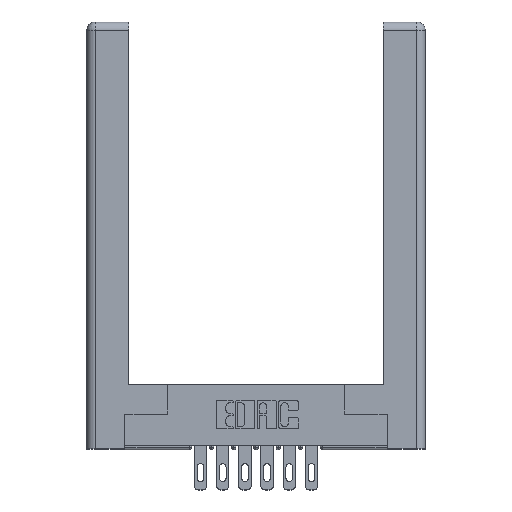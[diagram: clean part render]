
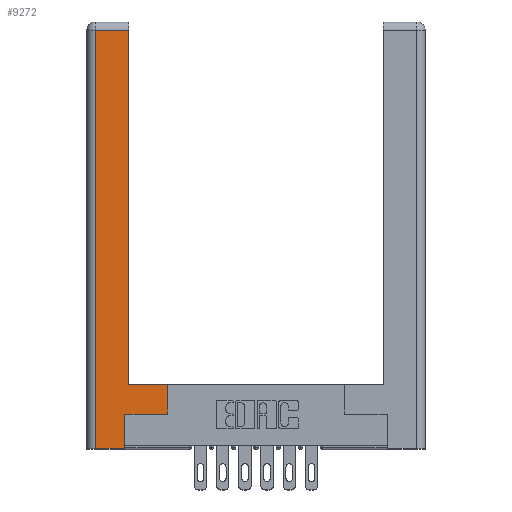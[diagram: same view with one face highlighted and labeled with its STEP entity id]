
A CAD part, top view. The second image highlights one B-rep face of the part: STEP entity #9272.
In plain terms, the highlighted planar face has unit normal (0, 0, 1).
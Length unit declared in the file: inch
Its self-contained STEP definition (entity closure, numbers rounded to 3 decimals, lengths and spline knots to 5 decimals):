
#87 = ORIENTED_EDGE ( 'NONE', *, *, #5223, .T. ) ;
#335 = ORIENTED_EDGE ( 'NONE', *, *, #5017, .T. ) ;
#490 = VECTOR ( 'NONE', #10808, 39.37008 ) ;
#1028 = CARTESIAN_POINT ( 'NONE',  ( 0.295, 3., 0. ) ) ;
#1227 = VECTOR ( 'NONE', #6869, 39.37008 ) ;
#1341 = CARTESIAN_POINT ( 'NONE',  ( 0.265, 0., 0. ) ) ;
#2209 = CARTESIAN_POINT ( 'NONE',  ( 0.0615, 0., 0. ) ) ;
#2702 = ORIENTED_EDGE ( 'NONE', *, *, #5107, .T. ) ;
#2739 = CARTESIAN_POINT ( 'NONE',  ( 0.565, 0.245, 0. ) ) ;
#3111 = CARTESIAN_POINT ( 'NONE',  ( 0.295, 0.45, 0. ) ) ;
#3531 = LINE ( 'NONE', #10332, #490 ) ;
#3705 = CARTESIAN_POINT ( 'NONE',  ( 0.295, 0.45, 0. ) ) ;
#3775 = LINE ( 'NONE', #5520, #8857 ) ;
#3804 = CARTESIAN_POINT ( 'NONE',  ( 0.0615, 2.94, 0. ) ) ;
#3820 = VERTEX_POINT ( 'NONE', #2209 ) ;
#3866 = FACE_OUTER_BOUND ( 'NONE', #8218, .T. ) ;
#4005 = VERTEX_POINT ( 'NONE', #3705 ) ;
#4191 = ORIENTED_EDGE ( 'NONE', *, *, #7445, .T. ) ;
#4548 = DIRECTION ( 'NONE',  ( -1., 0., 0. ) ) ;
#4716 = CARTESIAN_POINT ( 'NONE',  ( 0.295, 2.94, 0. ) ) ;
#4779 = AXIS2_PLACEMENT_3D ( 'NONE', #11039, #10870, #10853 ) ;
#5017 = EDGE_CURVE ( 'NONE', #3820, #8410, #3531, .T. ) ;
#5107 = EDGE_CURVE ( 'NONE', #12097, #4005, #12753, .T. ) ;
#5155 = VECTOR ( 'NONE', #4548, 39.37008 ) ;
#5193 = VERTEX_POINT ( 'NONE', #4716 ) ;
#5223 = EDGE_CURVE ( 'NONE', #4005, #5193, #8110, .T. ) ;
#5245 = EDGE_CURVE ( 'NONE', #5193, #6784, #10182, .T. ) ;
#5520 = CARTESIAN_POINT ( 'NONE',  ( 0.265, 0.245, 0. ) ) ;
#5847 = ORIENTED_EDGE ( 'NONE', *, *, #5245, .T. ) ;
#6556 = DIRECTION ( 'NONE',  ( 0., 1., 0. ) ) ;
#6784 = VERTEX_POINT ( 'NONE', #10791 ) ;
#6869 = DIRECTION ( 'NONE',  ( 1., 0., 0. ) ) ;
#6936 = VERTEX_POINT ( 'NONE', #6988 ) ;
#6988 = CARTESIAN_POINT ( 'NONE',  ( 0.565, 0.245, 0. ) ) ;
#7052 = VECTOR ( 'NONE', #7135, 39.37008 ) ;
#7135 = DIRECTION ( 'NONE',  ( 0., -1., 0. ) ) ;
#7342 = VECTOR ( 'NONE', #11834, 39.37008 ) ;
#7445 = EDGE_CURVE ( 'NONE', #6936, #12097, #12194, .T. ) ;
#7463 = CARTESIAN_POINT ( 'NONE',  ( 0.0615, 0., 0. ) ) ;
#8048 = ORIENTED_EDGE ( 'NONE', *, *, #9053, .T. ) ;
#8110 = LINE ( 'NONE', #1028, #12854 ) ;
#8218 = EDGE_LOOP ( 'NONE', ( #87, #5847, #8048, #335, #9637, #10563, #4191, #2702 ) ) ;
#8410 = VERTEX_POINT ( 'NONE', #1341 ) ;
#8743 = VERTEX_POINT ( 'NONE', #9324 ) ;
#8757 = CARTESIAN_POINT ( 'NONE',  ( 0.565, 0.45, 0. ) ) ;
#8857 = VECTOR ( 'NONE', #6556, 39.37008 ) ;
#9053 = EDGE_CURVE ( 'NONE', #6784, #3820, #9699, .T. ) ;
#9256 = LINE ( 'NONE', #2739, #1227 ) ;
#9272 = ADVANCED_FACE ( 'NONE', ( #3866 ), #10915, .F. ) ;
#9324 = CARTESIAN_POINT ( 'NONE',  ( 0.265, 0.245, 0. ) ) ;
#9637 = ORIENTED_EDGE ( 'NONE', *, *, #11997, .T. ) ;
#9699 = LINE ( 'NONE', #7463, #7052 ) ;
#10097 = EDGE_CURVE ( 'NONE', #8743, #6936, #9256, .T. ) ;
#10182 = LINE ( 'NONE', #3804, #5155 ) ;
#10255 = VECTOR ( 'NONE', #11257, 39.37008 ) ;
#10332 = CARTESIAN_POINT ( 'NONE',  ( 0.265, 0., 0. ) ) ;
#10563 = ORIENTED_EDGE ( 'NONE', *, *, #10097, .T. ) ;
#10791 = CARTESIAN_POINT ( 'NONE',  ( 0.0615, 2.94, 0. ) ) ;
#10808 = DIRECTION ( 'NONE',  ( 1., 0., 0. ) ) ;
#10853 = DIRECTION ( 'NONE',  ( -1., 0., 0. ) ) ;
#10870 = DIRECTION ( 'NONE',  ( 0., 0., -1. ) ) ;
#10915 = PLANE ( 'NONE',  #4779 ) ;
#11039 = CARTESIAN_POINT ( 'NONE',  ( 0., 0., 0. ) ) ;
#11083 = DIRECTION ( 'NONE',  ( 0., 1., 0. ) ) ;
#11211 = CARTESIAN_POINT ( 'NONE',  ( 0.565, 0.45, 0. ) ) ;
#11257 = DIRECTION ( 'NONE',  ( 0., 1., 0. ) ) ;
#11834 = DIRECTION ( 'NONE',  ( -1., 0., 0. ) ) ;
#11997 = EDGE_CURVE ( 'NONE', #8410, #8743, #3775, .T. ) ;
#12097 = VERTEX_POINT ( 'NONE', #8757 ) ;
#12194 = LINE ( 'NONE', #11211, #10255 ) ;
#12753 = LINE ( 'NONE', #3111, #7342 ) ;
#12854 = VECTOR ( 'NONE', #11083, 39.37008 ) ;
